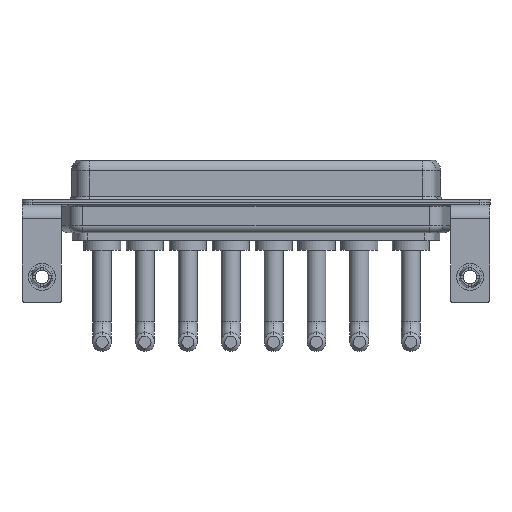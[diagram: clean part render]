
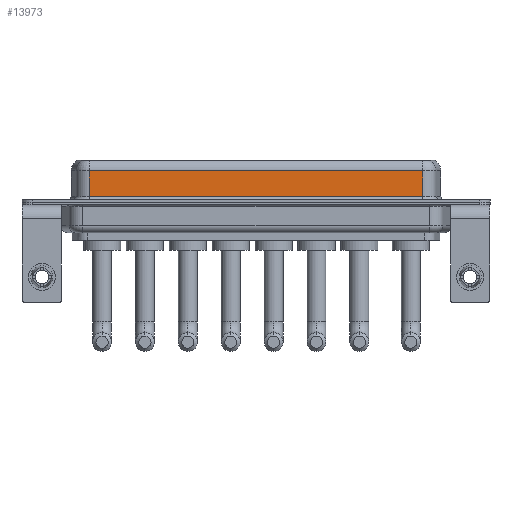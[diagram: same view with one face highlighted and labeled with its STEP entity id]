
A CAD part, front view. The second image highlights one B-rep face of the part: STEP entity #13973.
In plain terms, the highlighted planar face has unit normal (0, -1, 0).
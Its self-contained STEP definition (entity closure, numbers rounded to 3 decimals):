
#526 = EDGE_CURVE ( 'NONE', #3779, #14568, #5784, .T. ) ;
#544 = VECTOR ( 'NONE', #9949, 1000. ) ;
#1214 = EDGE_LOOP ( 'NONE', ( #2721, #4590, #1549, #6656 ) ) ;
#1454 = VECTOR ( 'NONE', #1936, 1000. ) ;
#1549 = ORIENTED_EDGE ( 'NONE', *, *, #526, .T. ) ;
#1936 = DIRECTION ( 'NONE',  ( 0., 0., -1. ) ) ;
#1991 = EDGE_CURVE ( 'NONE', #14568, #2391, #8220, .T. ) ;
#2016 = LINE ( 'NONE', #12783, #1454 ) ;
#2131 = DIRECTION ( 'NONE',  ( 1., 0., 0. ) ) ;
#2391 = VERTEX_POINT ( 'NONE', #2463 ) ;
#2463 = CARTESIAN_POINT ( 'NONE',  ( 56.462, -3.95, 0.9 ) ) ;
#2596 = CARTESIAN_POINT ( 'NONE',  ( 56.462, -3.95, 4.65 ) ) ;
#2721 = ORIENTED_EDGE ( 'NONE', *, *, #11088, .F. ) ;
#3779 = VERTEX_POINT ( 'NONE', #6720 ) ;
#4305 = AXIS2_PLACEMENT_3D ( 'NONE', #7024, #10384, #12828 ) ;
#4590 = ORIENTED_EDGE ( 'NONE', *, *, #15001, .T. ) ;
#5784 = LINE ( 'NONE', #5863, #11302 ) ;
#5863 = CARTESIAN_POINT ( 'NONE',  ( 7.038, -3.95, 6.4 ) ) ;
#6656 = ORIENTED_EDGE ( 'NONE', *, *, #1991, .T. ) ;
#6720 = CARTESIAN_POINT ( 'NONE',  ( 7.038, -3.95, 4.65 ) ) ;
#7024 = CARTESIAN_POINT ( 'NONE',  ( 56.462, -3.95, 6.4 ) ) ;
#8220 = LINE ( 'NONE', #14488, #8284 ) ;
#8284 = VECTOR ( 'NONE', #2131, 1000. ) ;
#9868 = CARTESIAN_POINT ( 'NONE',  ( 7.038, -3.95, 0.9 ) ) ;
#9949 = DIRECTION ( 'NONE',  ( -1., 0., 0. ) ) ;
#10384 = DIRECTION ( 'NONE',  ( 0., 1., 0. ) ) ;
#10455 = VERTEX_POINT ( 'NONE', #11226 ) ;
#11059 = LINE ( 'NONE', #2596, #544 ) ;
#11088 = EDGE_CURVE ( 'NONE', #10455, #2391, #2016, .T. ) ;
#11226 = CARTESIAN_POINT ( 'NONE',  ( 56.462, -3.95, 4.65 ) ) ;
#11302 = VECTOR ( 'NONE', #13213, 1000. ) ;
#12080 = PLANE ( 'NONE',  #4305 ) ;
#12783 = CARTESIAN_POINT ( 'NONE',  ( 56.462, -3.95, 6.4 ) ) ;
#12828 = DIRECTION ( 'NONE',  ( 0., 0., 1. ) ) ;
#13213 = DIRECTION ( 'NONE',  ( 0., 0., -1. ) ) ;
#13973 = ADVANCED_FACE ( 'NONE', ( #15669 ), #12080, .F. ) ;
#14488 = CARTESIAN_POINT ( 'NONE',  ( 56.462, -3.95, 0.9 ) ) ;
#14568 = VERTEX_POINT ( 'NONE', #9868 ) ;
#15001 = EDGE_CURVE ( 'NONE', #10455, #3779, #11059, .T. ) ;
#15669 = FACE_OUTER_BOUND ( 'NONE', #1214, .T. ) ;
